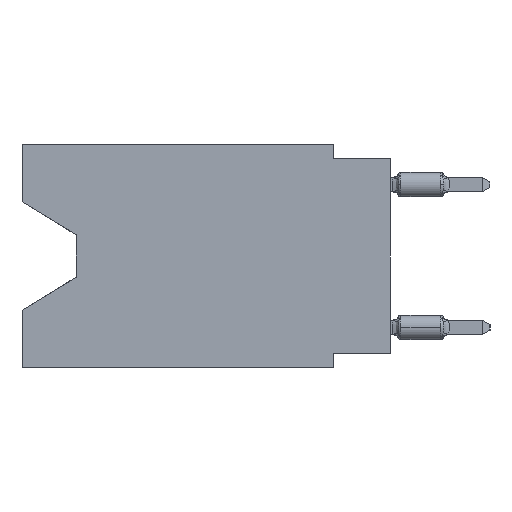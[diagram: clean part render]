
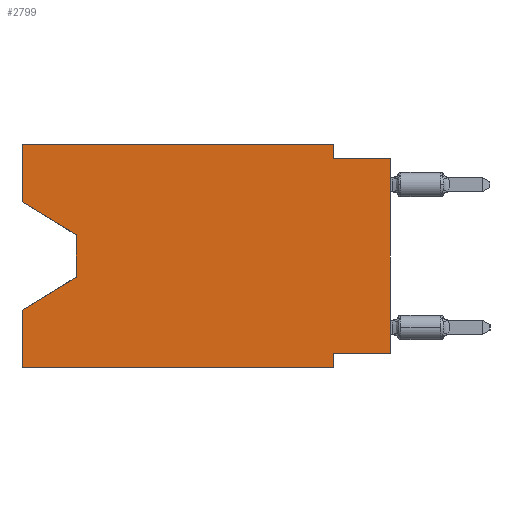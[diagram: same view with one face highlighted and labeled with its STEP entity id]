
A CAD part, left-side view. The second image highlights one B-rep face of the part: STEP entity #2799.
In plain terms, the highlighted planar face has unit normal (-1, 0, 0).
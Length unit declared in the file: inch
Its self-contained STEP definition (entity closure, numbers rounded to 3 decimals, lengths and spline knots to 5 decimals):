
#4 = CARTESIAN_POINT ( 'NONE',  ( 0., 0.55, -0.232 ) ) ;
#129 = EDGE_CURVE ( 'NONE', #10460, #24836, #15795, .T. ) ;
#256 = ORIENTED_EDGE ( 'NONE', *, *, #16060, .F. ) ;
#713 = DIRECTION ( 'NONE',  ( 0., 1., 0. ) ) ;
#854 = EDGE_CURVE ( 'NONE', #15006, #8602, #23562, .T. ) ;
#1309 = VECTOR ( 'NONE', #3815, 39.37008 ) ;
#1391 = VECTOR ( 'NONE', #19748, 39.37008 ) ;
#1887 = CARTESIAN_POINT ( 'NONE',  ( 0., 0.645, 0. ) ) ;
#2430 = EDGE_CURVE ( 'NONE', #15006, #18293, #22771, .T. ) ;
#2513 = DIRECTION ( 'NONE',  ( 0., -1., 0. ) ) ;
#2799 = ADVANCED_FACE ( 'NONE', ( #3853 ), #11794, .F. ) ;
#3069 = LINE ( 'NONE', #22890, #17792 ) ;
#3815 = DIRECTION ( 'NONE',  ( 0., -1., 0. ) ) ;
#3853 = FACE_OUTER_BOUND ( 'NONE', #20560, .T. ) ;
#4734 = LINE ( 'NONE', #16716, #16361 ) ;
#5361 = CARTESIAN_POINT ( 'NONE',  ( 0., 0.645, -0.39 ) ) ;
#5462 = CARTESIAN_POINT ( 'NONE',  ( 0., 0.645, -0.10025 ) ) ;
#5564 = LINE ( 'NONE', #19890, #1391 ) ;
#5613 = CARTESIAN_POINT ( 'NONE',  ( 0., 0.1, 0. ) ) ;
#5624 = CARTESIAN_POINT ( 'NONE',  ( 0., 0.645, 0. ) ) ;
#5753 = DIRECTION ( 'NONE',  ( 0., 0., 1. ) ) ;
#5756 = EDGE_CURVE ( 'NONE', #24695, #8880, #6336, .T. ) ;
#5808 = ORIENTED_EDGE ( 'NONE', *, *, #12871, .F. ) ;
#6108 = ORIENTED_EDGE ( 'NONE', *, *, #5756, .T. ) ;
#6336 = LINE ( 'NONE', #19894, #10105 ) ;
#6840 = LINE ( 'NONE', #14791, #17306 ) ;
#7919 = VERTEX_POINT ( 'NONE', #18768 ) ;
#8477 = CARTESIAN_POINT ( 'NONE',  ( 0., 0.1, -0.39 ) ) ;
#8602 = VERTEX_POINT ( 'NONE', #16348 ) ;
#8770 = CARTESIAN_POINT ( 'NONE',  ( 0., 0.1, -0.025 ) ) ;
#8880 = VERTEX_POINT ( 'NONE', #15299 ) ;
#9834 = DIRECTION ( 'NONE',  ( 0., 0., -1. ) ) ;
#9876 = LINE ( 'NONE', #15749, #19381 ) ;
#10105 = VECTOR ( 'NONE', #10383, 39.37008 ) ;
#10383 = DIRECTION ( 'NONE',  ( 0., 0.855, -0.519 ) ) ;
#10460 = VERTEX_POINT ( 'NONE', #5361 ) ;
#10470 = VERTEX_POINT ( 'NONE', #5613 ) ;
#10697 = VECTOR ( 'NONE', #25507, 39.37008 ) ;
#10857 = ORIENTED_EDGE ( 'NONE', *, *, #129, .T. ) ;
#10937 = ORIENTED_EDGE ( 'NONE', *, *, #15625, .F. ) ;
#11278 = AXIS2_PLACEMENT_3D ( 'NONE', #1887, #14006, #9834 ) ;
#11295 = ORIENTED_EDGE ( 'NONE', *, *, #13887, .F. ) ;
#11619 = EDGE_CURVE ( 'NONE', #8602, #24695, #17350, .T. ) ;
#11794 = PLANE ( 'NONE',  #11278 ) ;
#11867 = CARTESIAN_POINT ( 'NONE',  ( 0., 0.55, -0.158 ) ) ;
#12603 = DIRECTION ( 'NONE',  ( 0., 0., 1. ) ) ;
#12750 = CARTESIAN_POINT ( 'NONE',  ( 0., 0., -0.025 ) ) ;
#12871 = EDGE_CURVE ( 'NONE', #10460, #8880, #25451, .T. ) ;
#13887 = EDGE_CURVE ( 'NONE', #10470, #16062, #9876, .T. ) ;
#13979 = ORIENTED_EDGE ( 'NONE', *, *, #11619, .T. ) ;
#14006 = DIRECTION ( 'NONE',  ( 1., 0., 0. ) ) ;
#14152 = VERTEX_POINT ( 'NONE', #12750 ) ;
#14261 = EDGE_CURVE ( 'NONE', #7919, #14152, #21595, .T. ) ;
#14432 = VECTOR ( 'NONE', #5753, 39.37008 ) ;
#14538 = DIRECTION ( 'NONE',  ( 0., 0., -1. ) ) ;
#14791 = CARTESIAN_POINT ( 'NONE',  ( 0., 0., -0.365 ) ) ;
#15006 = VERTEX_POINT ( 'NONE', #5462 ) ;
#15299 = CARTESIAN_POINT ( 'NONE',  ( 0., 0.645, -0.28975 ) ) ;
#15486 = DIRECTION ( 'NONE',  ( 0., -0.855, -0.519 ) ) ;
#15625 = EDGE_CURVE ( 'NONE', #24596, #24836, #3069, .T. ) ;
#15749 = CARTESIAN_POINT ( 'NONE',  ( 0., 0.1, 0. ) ) ;
#15795 = LINE ( 'NONE', #21667, #1309 ) ;
#16060 = EDGE_CURVE ( 'NONE', #16062, #14152, #4734, .T. ) ;
#16062 = VERTEX_POINT ( 'NONE', #8770 ) ;
#16348 = CARTESIAN_POINT ( 'NONE',  ( 0., 0.55, -0.158 ) ) ;
#16351 = ORIENTED_EDGE ( 'NONE', *, *, #16701, .F. ) ;
#16361 = VECTOR ( 'NONE', #2513, 39.37008 ) ;
#16580 = ORIENTED_EDGE ( 'NONE', *, *, #14261, .T. ) ;
#16672 = ORIENTED_EDGE ( 'NONE', *, *, #2430, .F. ) ;
#16701 = EDGE_CURVE ( 'NONE', #18293, #10470, #5564, .T. ) ;
#16716 = CARTESIAN_POINT ( 'NONE',  ( 0., 0., -0.025 ) ) ;
#17306 = VECTOR ( 'NONE', #713, 39.37008 ) ;
#17350 = LINE ( 'NONE', #11867, #20215 ) ;
#17725 = VECTOR ( 'NONE', #15486, 39.37008 ) ;
#17792 = VECTOR ( 'NONE', #14538, 39.37008 ) ;
#18293 = VERTEX_POINT ( 'NONE', #24245 ) ;
#18768 = CARTESIAN_POINT ( 'NONE',  ( 0., 0., -0.365 ) ) ;
#19133 = VECTOR ( 'NONE', #12603, 39.37008 ) ;
#19163 = EDGE_CURVE ( 'NONE', #7919, #24596, #6840, .T. ) ;
#19381 = VECTOR ( 'NONE', #23447, 39.37008 ) ;
#19748 = DIRECTION ( 'NONE',  ( 0., -1., 0. ) ) ;
#19890 = CARTESIAN_POINT ( 'NONE',  ( 0., 0.645, 0. ) ) ;
#19894 = CARTESIAN_POINT ( 'NONE',  ( 0., 0.55, -0.232 ) ) ;
#20215 = VECTOR ( 'NONE', #25323, 39.37008 ) ;
#20295 = CARTESIAN_POINT ( 'NONE',  ( 0., 0.645, 0. ) ) ;
#20560 = EDGE_LOOP ( 'NONE', ( #22873, #13979, #6108, #5808, #10857, #10937, #21576, #16580, #256, #11295, #16351, #16672 ) ) ;
#21576 = ORIENTED_EDGE ( 'NONE', *, *, #19163, .F. ) ;
#21595 = LINE ( 'NONE', #23290, #10697 ) ;
#21667 = CARTESIAN_POINT ( 'NONE',  ( 0., 0.645, -0.39 ) ) ;
#22771 = LINE ( 'NONE', #20295, #19133 ) ;
#22873 = ORIENTED_EDGE ( 'NONE', *, *, #854, .T. ) ;
#22890 = CARTESIAN_POINT ( 'NONE',  ( 0., 0.1, -0.39 ) ) ;
#23290 = CARTESIAN_POINT ( 'NONE',  ( 0., 0., 0. ) ) ;
#23437 = CARTESIAN_POINT ( 'NONE',  ( 0., 0.645, -0.10025 ) ) ;
#23447 = DIRECTION ( 'NONE',  ( 0., 0., -1. ) ) ;
#23562 = LINE ( 'NONE', #23437, #17725 ) ;
#23877 = CARTESIAN_POINT ( 'NONE',  ( 0., 0.1, -0.365 ) ) ;
#24245 = CARTESIAN_POINT ( 'NONE',  ( 0., 0.645, 0. ) ) ;
#24596 = VERTEX_POINT ( 'NONE', #23877 ) ;
#24695 = VERTEX_POINT ( 'NONE', #4 ) ;
#24836 = VERTEX_POINT ( 'NONE', #8477 ) ;
#25323 = DIRECTION ( 'NONE',  ( 0., 0., -1. ) ) ;
#25451 = LINE ( 'NONE', #5624, #14432 ) ;
#25507 = DIRECTION ( 'NONE',  ( 0., 0., 1. ) ) ;
